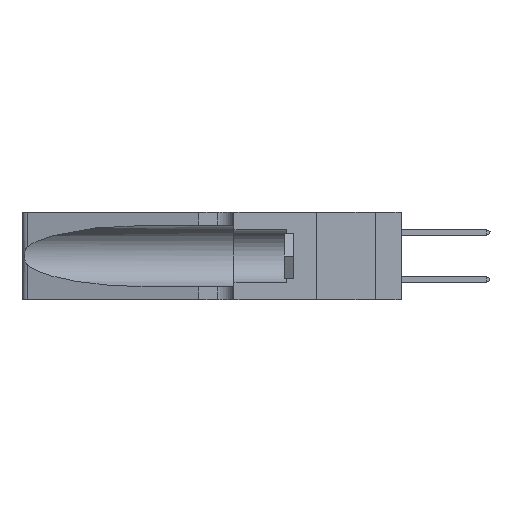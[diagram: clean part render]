
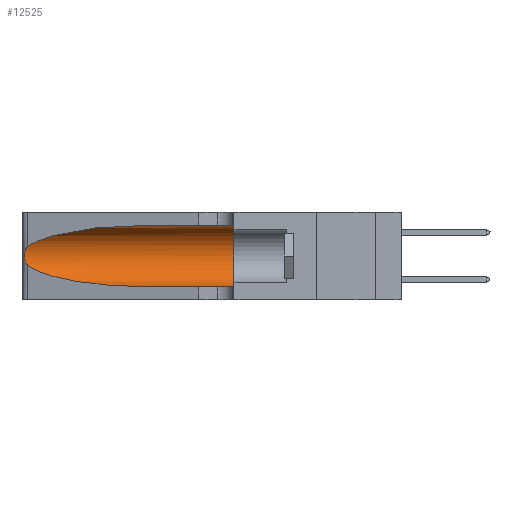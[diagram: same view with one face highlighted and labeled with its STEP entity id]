
A CAD part, left-side view. The second image highlights one B-rep face of the part: STEP entity #12525.
In plain terms, the highlighted cylindrical face has radius 3.308 mm (diameter 6.617 mm), a partial arc.
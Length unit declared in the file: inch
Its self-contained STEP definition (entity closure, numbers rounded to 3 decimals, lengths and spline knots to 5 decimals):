
#653 = VERTEX_POINT ( 'NONE', #20790 ) ;
#1225 = CARTESIAN_POINT ( 'NONE',  ( 0.1305, 1.61858, 0.185 ) ) ;
#1285 = CARTESIAN_POINT ( 'NONE',  ( 0.25789, 1.23486, 0.15765 ) ) ;
#2287 = LINE ( 'NONE', #19196, #23665 ) ;
#2609 = CARTESIAN_POINT ( 'NONE',  ( 0.2373, 1.15595, 0.28018 ) ) ;
#3092 = DIRECTION ( 'NONE',  ( 0., 1., 0. ) ) ;
#3315 = CARTESIAN_POINT ( 'NONE',  ( 0.25555, 1.22994, 0.2215 ) ) ;
#3405 = CARTESIAN_POINT ( 'NONE',  ( 0.25555, 1.22993, 0.14849 ) ) ;
#5494 = EDGE_CURVE ( 'NONE', #11925, #17663, #12217, .T. ) ;
#5536 = DIRECTION ( 'NONE',  ( 0., -1., 0. ) ) ;
#6398 = ORIENTED_EDGE ( 'NONE', *, *, #9911, .T. ) ;
#6680 = CYLINDRICAL_SURFACE ( 'NONE', #7738, 0.13025 ) ;
#7050 = VERTEX_POINT ( 'NONE', #23616 ) ;
#7282 = CARTESIAN_POINT ( 'NONE',  ( 0.1305, 0.72297, 0.05475 ) ) ;
#7354 = FACE_OUTER_BOUND ( 'NONE', #20905, .T. ) ;
#7526 = CARTESIAN_POINT ( 'NONE',  ( 0.25787, 1.23484, 0.2124 ) ) ;
#7737 = CARTESIAN_POINT ( 'NONE',  ( 0.25487, 1.22718, 0.14631 ) ) ;
#7738 = AXIS2_PLACEMENT_3D ( 'NONE', #1225, #15881, #15785 ) ;
#8547 = ORIENTED_EDGE ( 'NONE', *, *, #25895, .T. ) ;
#8576 = CARTESIAN_POINT ( 'NONE',  ( 0.1305, 0.72297, 0.05475 ) ) ;
#8736 = CARTESIAN_POINT ( 'NONE',  ( 0.1305, 0.35, 0.31525 ) ) ;
#9593 = CARTESIAN_POINT ( 'NONE',  ( 0.26018, 1.23835, 0.19895 ) ) ;
#9911 = EDGE_CURVE ( 'NONE', #25838, #7050, #19831, .T. ) ;
#11128 = AXIS2_PLACEMENT_3D ( 'NONE', #15526, #3092, #17606 ) ;
#11664 = CARTESIAN_POINT ( 'NONE',  ( 0.26075, 1.23896, 0.178 ) ) ;
#11925 = VERTEX_POINT ( 'NONE', #14237 ) ;
#12217 = B_SPLINE_CURVE_WITH_KNOTS ( 'NONE', 3,
 ( #17822, #3315, #19857, #7526, #21952, #9593, #24026, #11664, #26094, #13751, #1285, #15849, #3405, #17915 ),
 .UNSPECIFIED., .F., .F.,
 ( 4, 2, 2, 2, 2, 2, 4 ),
 ( 0., 0.00027, 0.00053, 0.00107, 0.0016, 0.00187, 0.00214 ),
 .UNSPECIFIED. ) ;
#12525 = ADVANCED_FACE ( 'NONE', ( #7354 ), #6680, .F. ) ;
#12671 = ORIENTED_EDGE ( 'NONE', *, *, #25304, .F. ) ;
#12961 = CARTESIAN_POINT ( 'NONE',  ( 0.18966, 0.96281, 0.31525 ) ) ;
#13751 = CARTESIAN_POINT ( 'NONE',  ( 0.25856, 1.23593, 0.16098 ) ) ;
#14237 = CARTESIAN_POINT ( 'NONE',  ( 0.25487, 1.22718, 0.22369 ) ) ;
#14258 = CIRCLE ( 'NONE', #11128, 0.13025 ) ;
#14370 = VECTOR ( 'NONE', #5536, 39.37008 ) ;
#14438 = ORIENTED_EDGE ( 'NONE', *, *, #5494, .T. ) ;
#15019 =( BOUNDED_CURVE ( )  B_SPLINE_CURVE ( 3, ( #15520, #17595, #19638, #7282 ),
 .UNSPECIFIED., .F., .F. ) 
 B_SPLINE_CURVE_WITH_KNOTS ( ( 4, 4 ),
 ( 3.44316, 4.71239 ),
 .UNSPECIFIED. ) 
 CURVE ( )  GEOMETRIC_REPRESENTATION_ITEM ( )  RATIONAL_B_SPLINE_CURVE ( ( 1., 0.87, 0.87, 1. ) ) 
 REPRESENTATION_ITEM ( '' )  );
#15520 = CARTESIAN_POINT ( 'NONE',  ( 0.25487, 1.22718, 0.14631 ) ) ;
#15526 = CARTESIAN_POINT ( 'NONE',  ( 0.1305, 0.35, 0.185 ) ) ;
#15785 = DIRECTION ( 'NONE',  ( 0., 0., -1. ) ) ;
#15849 = CARTESIAN_POINT ( 'NONE',  ( 0.25639, 1.23186, 0.15144 ) ) ;
#15881 = DIRECTION ( 'NONE',  ( 0., -1., 0. ) ) ;
#15892 = CARTESIAN_POINT ( 'NONE',  ( 0.1305, 1.61858, 0.05475 ) ) ;
#17137 = CARTESIAN_POINT ( 'NONE',  ( 0.25487, 1.22718, 0.22369 ) ) ;
#17595 = CARTESIAN_POINT ( 'NONE',  ( 0.2373, 1.15595, 0.08982 ) ) ;
#17606 = DIRECTION ( 'NONE',  ( 0., 0., 1. ) ) ;
#17663 = VERTEX_POINT ( 'NONE', #7737 ) ;
#17822 = CARTESIAN_POINT ( 'NONE',  ( 0.25487, 1.22718, 0.22369 ) ) ;
#17852 =( BOUNDED_CURVE ( )  B_SPLINE_CURVE ( 3, ( #23249, #12961, #2609, #17137 ),
 .UNSPECIFIED., .F., .F. ) 
 B_SPLINE_CURVE_WITH_KNOTS ( ( 4, 4 ),
 ( 1.5708, 2.84003 ),
 .UNSPECIFIED. ) 
 CURVE ( )  GEOMETRIC_REPRESENTATION_ITEM ( )  RATIONAL_B_SPLINE_CURVE ( ( 1., 0.87, 0.87, 1. ) ) 
 REPRESENTATION_ITEM ( '' )  );
#17915 = CARTESIAN_POINT ( 'NONE',  ( 0.25487, 1.22718, 0.14631 ) ) ;
#18062 = ORIENTED_EDGE ( 'NONE', *, *, #19951, .T. ) ;
#19196 = CARTESIAN_POINT ( 'NONE',  ( 0.1305, 1.61858, 0.31525 ) ) ;
#19638 = CARTESIAN_POINT ( 'NONE',  ( 0.18966, 0.96281, 0.05475 ) ) ;
#19831 = LINE ( 'NONE', #15892, #14370 ) ;
#19857 = CARTESIAN_POINT ( 'NONE',  ( 0.25639, 1.23184, 0.21858 ) ) ;
#19951 = EDGE_CURVE ( 'NONE', #17663, #25838, #15019, .T. ) ;
#20790 = CARTESIAN_POINT ( 'NONE',  ( 0.1305, 0.72297, 0.31525 ) ) ;
#20905 = EDGE_LOOP ( 'NONE', ( #8547, #14438, #18062, #6398, #21949, #12671 ) ) ;
#21949 = ORIENTED_EDGE ( 'NONE', *, *, #22342, .F. ) ;
#21952 = CARTESIAN_POINT ( 'NONE',  ( 0.25854, 1.2359, 0.20912 ) ) ;
#22342 = EDGE_CURVE ( 'NONE', #22810, #7050, #14258, .T. ) ;
#22810 = VERTEX_POINT ( 'NONE', #8736 ) ;
#23249 = CARTESIAN_POINT ( 'NONE',  ( 0.1305, 0.72297, 0.31525 ) ) ;
#23362 = DIRECTION ( 'NONE',  ( 0., -1., 0. ) ) ;
#23616 = CARTESIAN_POINT ( 'NONE',  ( 0.1305, 0.35, 0.05475 ) ) ;
#23665 = VECTOR ( 'NONE', #23362, 39.37008 ) ;
#24026 = CARTESIAN_POINT ( 'NONE',  ( 0.26075, 1.23896, 0.19203 ) ) ;
#25304 = EDGE_CURVE ( 'NONE', #653, #22810, #2287, .T. ) ;
#25838 = VERTEX_POINT ( 'NONE', #8576 ) ;
#25895 = EDGE_CURVE ( 'NONE', #653, #11925, #17852, .T. ) ;
#26094 = CARTESIAN_POINT ( 'NONE',  ( 0.26017, 1.23833, 0.17102 ) ) ;
